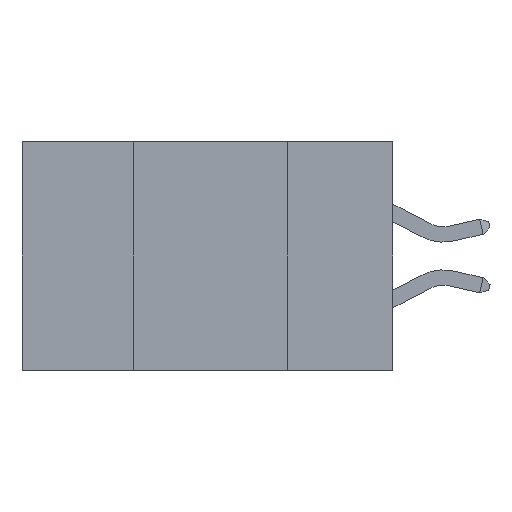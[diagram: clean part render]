
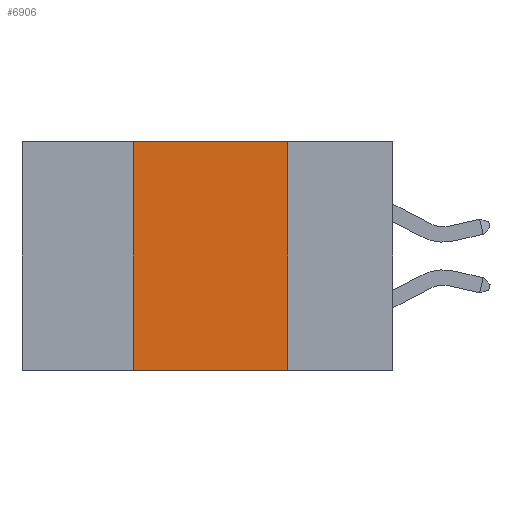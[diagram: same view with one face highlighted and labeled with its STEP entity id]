
A CAD part, left-side view. The second image highlights one B-rep face of the part: STEP entity #6906.
In plain terms, the highlighted planar face has unit normal (-1, 0, 0).
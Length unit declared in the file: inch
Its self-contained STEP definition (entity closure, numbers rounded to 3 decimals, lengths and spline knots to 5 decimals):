
#1676 = VECTOR ( 'NONE', #6042, 39.37008 ) ;
#2080 = VERTEX_POINT ( 'NONE', #21514 ) ;
#2746 = AXIS2_PLACEMENT_3D ( 'NONE', #11934, #15788, #13902 ) ;
#3323 = CARTESIAN_POINT ( 'NONE',  ( 0., 0.42, 0. ) ) ;
#5146 = CARTESIAN_POINT ( 'NONE',  ( 0., 0.6, 0. ) ) ;
#5910 = ORIENTED_EDGE ( 'NONE', *, *, #14405, .T. ) ;
#6042 = DIRECTION ( 'NONE',  ( 0., 0., -1. ) ) ;
#6906 = ADVANCED_FACE ( 'NONE', ( #15609 ), #21589, .F. ) ;
#7466 = VERTEX_POINT ( 'NONE', #10473 ) ;
#8938 = VERTEX_POINT ( 'NONE', #10957 ) ;
#9105 = DIRECTION ( 'NONE',  ( 0., -1., 0. ) ) ;
#9109 = CARTESIAN_POINT ( 'NONE',  ( 0., 0.42, 0. ) ) ;
#9683 = VERTEX_POINT ( 'NONE', #3323 ) ;
#9745 = VECTOR ( 'NONE', #10860, 39.37008 ) ;
#10062 = EDGE_LOOP ( 'NONE', ( #19884, #21604, #18487, #5910 ) ) ;
#10091 = VECTOR ( 'NONE', #16985, 39.37008 ) ;
#10473 = CARTESIAN_POINT ( 'NONE',  ( 0., 0.17, 0. ) ) ;
#10860 = DIRECTION ( 'NONE',  ( 0., 0., 1. ) ) ;
#10957 = CARTESIAN_POINT ( 'NONE',  ( 0., 0.42, -0.37 ) ) ;
#11644 = EDGE_CURVE ( 'NONE', #9683, #7466, #18406, .T. ) ;
#11934 = CARTESIAN_POINT ( 'NONE',  ( 0., 0.6, 0. ) ) ;
#13902 = DIRECTION ( 'NONE',  ( 0., 0., -1. ) ) ;
#14405 = EDGE_CURVE ( 'NONE', #8938, #2080, #18081, .T. ) ;
#15609 = FACE_OUTER_BOUND ( 'NONE', #10062, .T. ) ;
#15788 = DIRECTION ( 'NONE',  ( 1., 0., 0. ) ) ;
#16258 = EDGE_CURVE ( 'NONE', #8938, #9683, #18640, .T. ) ;
#16985 = DIRECTION ( 'NONE',  ( 0., -1., 0. ) ) ;
#17388 = LINE ( 'NONE', #21668, #1676 ) ;
#18081 = LINE ( 'NONE', #19124, #10091 ) ;
#18406 = LINE ( 'NONE', #5146, #22167 ) ;
#18487 = ORIENTED_EDGE ( 'NONE', *, *, #16258, .F. ) ;
#18640 = LINE ( 'NONE', #9109, #9745 ) ;
#19124 = CARTESIAN_POINT ( 'NONE',  ( 0., 0.6, -0.37 ) ) ;
#19884 = ORIENTED_EDGE ( 'NONE', *, *, #24163, .F. ) ;
#21514 = CARTESIAN_POINT ( 'NONE',  ( 0., 0.17, -0.37 ) ) ;
#21589 = PLANE ( 'NONE',  #2746 ) ;
#21604 = ORIENTED_EDGE ( 'NONE', *, *, #11644, .F. ) ;
#21668 = CARTESIAN_POINT ( 'NONE',  ( 0., 0.17, 0. ) ) ;
#22167 = VECTOR ( 'NONE', #9105, 39.37008 ) ;
#24163 = EDGE_CURVE ( 'NONE', #7466, #2080, #17388, .T. ) ;
